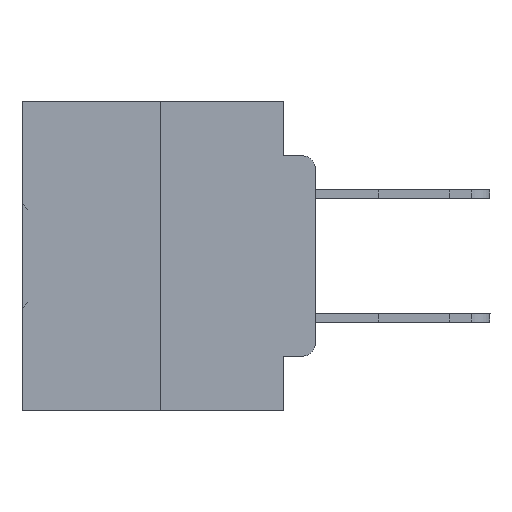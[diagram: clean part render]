
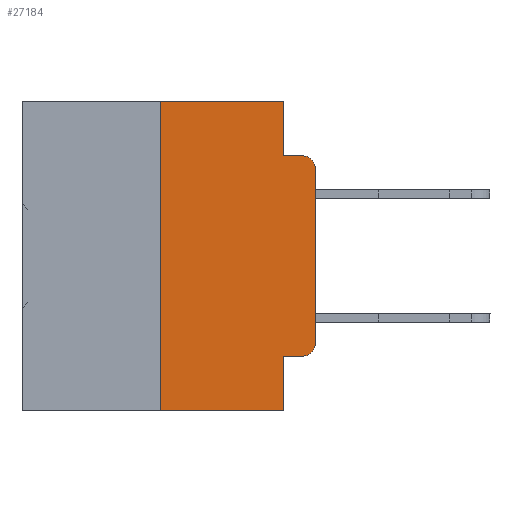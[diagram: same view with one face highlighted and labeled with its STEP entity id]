
A CAD part, left-side view. The second image highlights one B-rep face of the part: STEP entity #27184.
In plain terms, the highlighted planar face has unit normal (-1, 0, 0).
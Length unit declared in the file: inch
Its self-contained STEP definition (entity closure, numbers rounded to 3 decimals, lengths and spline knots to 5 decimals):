
#59 = CARTESIAN_POINT ( 'NONE',  ( 0., 0.02, -0.3915 ) ) ;
#401 = DIRECTION ( 'NONE',  ( -1., 0., 0. ) ) ;
#726 = VERTEX_POINT ( 'NONE', #18766 ) ;
#738 = EDGE_LOOP ( 'NONE', ( #14356, #32108, #16212, #23273, #22139, #34574, #29364, #14367, #1657, #23614 ) ) ;
#995 = CARTESIAN_POINT ( 'NONE',  ( 0., 0., -0.1085 ) ) ;
#1472 = CARTESIAN_POINT ( 'NONE',  ( 0., 0.25, 0. ) ) ;
#1636 = CARTESIAN_POINT ( 'NONE',  ( 0., 0.051, -0.4115 ) ) ;
#1657 = ORIENTED_EDGE ( 'NONE', *, *, #21756, .T. ) ;
#1982 = DIRECTION ( 'NONE',  ( -1., 0., 0. ) ) ;
#2890 = LINE ( 'NONE', #3826, #22521 ) ;
#3209 = AXIS2_PLACEMENT_3D ( 'NONE', #36320, #1982, #4872 ) ;
#3826 = CARTESIAN_POINT ( 'NONE',  ( 0., 0.25, 0. ) ) ;
#4872 = DIRECTION ( 'NONE',  ( 0., 0., -1. ) ) ;
#4999 = DIRECTION ( 'NONE',  ( 0., 0., -1. ) ) ;
#5564 = EDGE_CURVE ( 'NONE', #29751, #31294, #22101, .T. ) ;
#5664 = EDGE_CURVE ( 'NONE', #33419, #25328, #2890, .T. ) ;
#7097 = CARTESIAN_POINT ( 'NONE',  ( 0., 0.473, 0. ) ) ;
#7253 = LINE ( 'NONE', #11615, #32714 ) ;
#8567 = AXIS2_PLACEMENT_3D ( 'NONE', #27132, #32595, #21583 ) ;
#8763 = FACE_OUTER_BOUND ( 'NONE', #738, .T. ) ;
#9864 = PLANE ( 'NONE',  #8567 ) ;
#11044 = CARTESIAN_POINT ( 'NONE',  ( 0., 0.02, -0.4115 ) ) ;
#11560 = VERTEX_POINT ( 'NONE', #11864 ) ;
#11615 = CARTESIAN_POINT ( 'NONE',  ( 0., 0.051, 0. ) ) ;
#11662 = DIRECTION ( 'NONE',  ( 0., 0., -1. ) ) ;
#11864 = CARTESIAN_POINT ( 'NONE',  ( 0., 0.051, -0.4115 ) ) ;
#12270 = CIRCLE ( 'NONE', #3209, 0.02 ) ;
#12759 = CARTESIAN_POINT ( 'NONE',  ( 0., 0.051, -0.0885 ) ) ;
#12828 = EDGE_CURVE ( 'NONE', #31294, #726, #12270, .T. ) ;
#13155 = CARTESIAN_POINT ( 'NONE',  ( 0., 0.473, -0.5 ) ) ;
#13164 = VECTOR ( 'NONE', #16244, 39.37008 ) ;
#13500 = DIRECTION ( 'NONE',  ( 0., -1., 0. ) ) ;
#13580 = EDGE_CURVE ( 'NONE', #25328, #17991, #27926, .T. ) ;
#14356 = ORIENTED_EDGE ( 'NONE', *, *, #5564, .T. ) ;
#14367 = ORIENTED_EDGE ( 'NONE', *, *, #14573, .F. ) ;
#14573 = EDGE_CURVE ( 'NONE', #11560, #29570, #7253, .T. ) ;
#14634 = DIRECTION ( 'NONE',  ( 0., 0., -1. ) ) ;
#15955 = DIRECTION ( 'NONE',  ( 0., 0., 1. ) ) ;
#16212 = ORIENTED_EDGE ( 'NONE', *, *, #24582, .F. ) ;
#16244 = DIRECTION ( 'NONE',  ( 0., -1., 0. ) ) ;
#16545 = CARTESIAN_POINT ( 'NONE',  ( 0., 0.051, 0. ) ) ;
#17429 = EDGE_CURVE ( 'NONE', #33419, #29570, #35932, .T. ) ;
#17808 = DIRECTION ( 'NONE',  ( 0., 0., 1. ) ) ;
#17991 = VERTEX_POINT ( 'NONE', #16545 ) ;
#18766 = CARTESIAN_POINT ( 'NONE',  ( 0., 0.02, -0.0885 ) ) ;
#19215 = EDGE_CURVE ( 'NONE', #17991, #31255, #19564, .T. ) ;
#19462 = VECTOR ( 'NONE', #15955, 39.37008 ) ;
#19564 = LINE ( 'NONE', #30741, #28917 ) ;
#21583 = DIRECTION ( 'NONE',  ( 0., 0., -1. ) ) ;
#21756 = EDGE_CURVE ( 'NONE', #11560, #30971, #27467, .T. ) ;
#22101 = LINE ( 'NONE', #30062, #19462 ) ;
#22139 = ORIENTED_EDGE ( 'NONE', *, *, #13580, .F. ) ;
#22521 = VECTOR ( 'NONE', #17808, 39.37008 ) ;
#22744 = VECTOR ( 'NONE', #34837, 39.37008 ) ;
#23273 = ORIENTED_EDGE ( 'NONE', *, *, #19215, .F. ) ;
#23614 = ORIENTED_EDGE ( 'NONE', *, *, #28121, .T. ) ;
#24582 = EDGE_CURVE ( 'NONE', #31255, #726, #29450, .T. ) ;
#25328 = VERTEX_POINT ( 'NONE', #1472 ) ;
#27132 = CARTESIAN_POINT ( 'NONE',  ( 0., 0.473, 0. ) ) ;
#27184 = ADVANCED_FACE ( 'NONE', ( #8763 ), #9864, .F. ) ;
#27467 = LINE ( 'NONE', #1636, #13164 ) ;
#27584 = CIRCLE ( 'NONE', #31557, 0.02 ) ;
#27847 = CARTESIAN_POINT ( 'NONE',  ( 0., 0., -0.3915 ) ) ;
#27926 = LINE ( 'NONE', #7097, #31468 ) ;
#28121 = EDGE_CURVE ( 'NONE', #30971, #29751, #27584, .T. ) ;
#28917 = VECTOR ( 'NONE', #4999, 39.37008 ) ;
#29364 = ORIENTED_EDGE ( 'NONE', *, *, #17429, .T. ) ;
#29450 = LINE ( 'NONE', #35097, #22744 ) ;
#29541 = CARTESIAN_POINT ( 'NONE',  ( 0., 0.25, -0.5 ) ) ;
#29570 = VERTEX_POINT ( 'NONE', #32932 ) ;
#29751 = VERTEX_POINT ( 'NONE', #27847 ) ;
#30062 = CARTESIAN_POINT ( 'NONE',  ( 0., 0., 0. ) ) ;
#30741 = CARTESIAN_POINT ( 'NONE',  ( 0., 0.051, 0. ) ) ;
#30971 = VERTEX_POINT ( 'NONE', #11044 ) ;
#31255 = VERTEX_POINT ( 'NONE', #12759 ) ;
#31294 = VERTEX_POINT ( 'NONE', #995 ) ;
#31468 = VECTOR ( 'NONE', #13500, 39.37008 ) ;
#31557 = AXIS2_PLACEMENT_3D ( 'NONE', #59, #401, #11662 ) ;
#31883 = VECTOR ( 'NONE', #36355, 39.37008 ) ;
#32108 = ORIENTED_EDGE ( 'NONE', *, *, #12828, .T. ) ;
#32595 = DIRECTION ( 'NONE',  ( 1., 0., 0. ) ) ;
#32714 = VECTOR ( 'NONE', #14634, 39.37008 ) ;
#32932 = CARTESIAN_POINT ( 'NONE',  ( 0., 0.051, -0.5 ) ) ;
#33419 = VERTEX_POINT ( 'NONE', #29541 ) ;
#34574 = ORIENTED_EDGE ( 'NONE', *, *, #5664, .F. ) ;
#34837 = DIRECTION ( 'NONE',  ( 0., -1., 0. ) ) ;
#35097 = CARTESIAN_POINT ( 'NONE',  ( 0., 0.051, -0.0885 ) ) ;
#35932 = LINE ( 'NONE', #13155, #31883 ) ;
#36320 = CARTESIAN_POINT ( 'NONE',  ( 0., 0.02, -0.1085 ) ) ;
#36355 = DIRECTION ( 'NONE',  ( 0., -1., 0. ) ) ;
